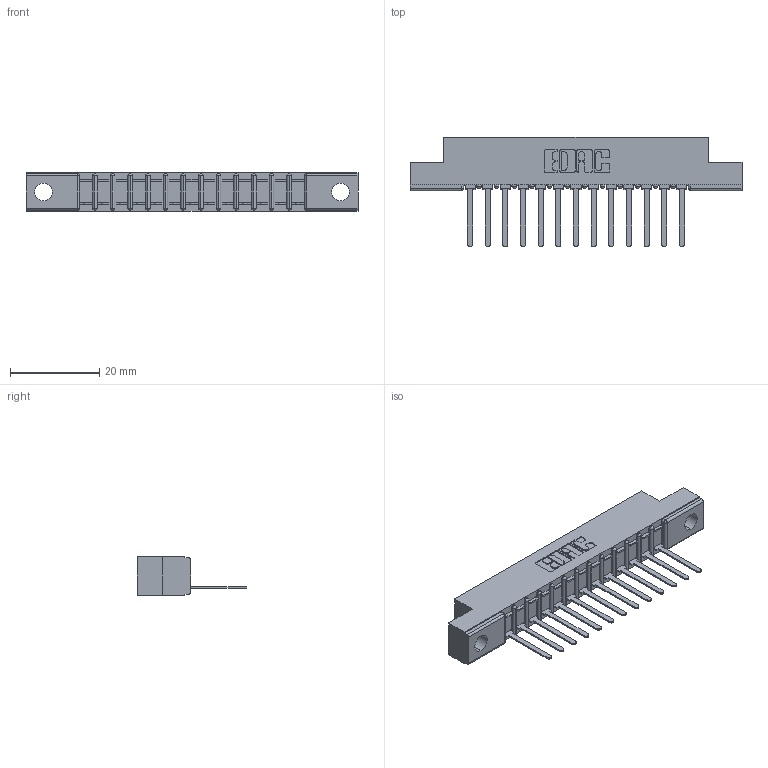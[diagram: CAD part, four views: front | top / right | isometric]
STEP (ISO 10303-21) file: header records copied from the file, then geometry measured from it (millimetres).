
FILE_DESCRIPTION (( 'STEP AP203' ), '1' );
FILE_NAME ('357-013-541-104.STEP', '2018-08-07T23:03:08', ( '' ), ( '' ), 'SwSTEP 2.0', 'SolidWorks 2016', '' );
FILE_SCHEMA (( 'CONFIG_CONTROL_DESIGN' ));
Length unit declared in the file: inch
Products named in the file (3): 307 Part_.156 Dia Mounting Holes; 307-290-002_541; 357-013-541-104
Assembly tree (14 placements, depth 2):
  357-013-541-104
    307 Part_.156 Dia Mounting Holes
    307-290-002_541  x13
Bounding box: 74.52 x 24.59 x 8.71 mm (x, y, z)
Volume: 4845.9 mm3; surface area: 8425.8 mm2
Topology: 14 solids, 14 shells, 1108 faces, 3375 edges, 2210 vertices
Faces by surface type: plane 669, cylinder 411, sphere 28
Entity records: 15856 total; most frequent: CARTESIAN_POINT 2674, ORIENTED_EDGE 2662, DIRECTION 2603, EDGE_CURVE 1331, VECTOR 1013, LINE 1013, VERTEX_POINT 866, AXIS2_PLACEMENT_3D 795
